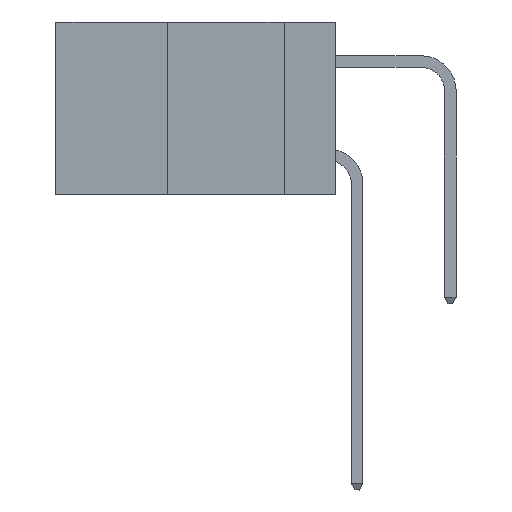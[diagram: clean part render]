
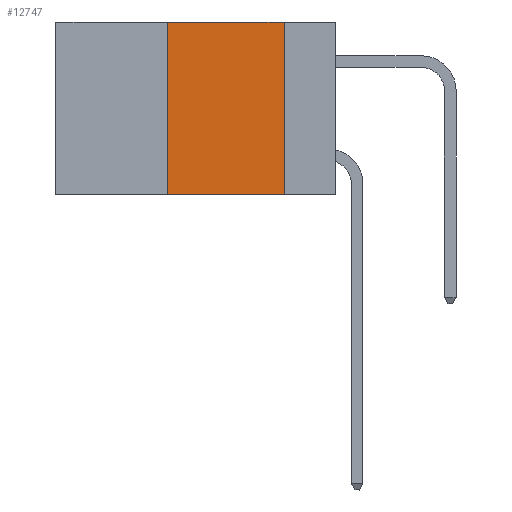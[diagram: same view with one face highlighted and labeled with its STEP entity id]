
A CAD part, left-side view. The second image highlights one B-rep face of the part: STEP entity #12747.
In plain terms, the highlighted planar face has unit normal (-1, 0, 0).
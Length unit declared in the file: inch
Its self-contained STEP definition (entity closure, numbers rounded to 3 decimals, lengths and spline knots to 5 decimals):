
#814 = CARTESIAN_POINT ( 'NONE',  ( 0., 0.36, 0. ) ) ;
#1652 = DIRECTION ( 'NONE',  ( 1., 0., 0. ) ) ;
#2081 = DIRECTION ( 'NONE',  ( 0., 0., 1. ) ) ;
#2251 = VERTEX_POINT ( 'NONE', #4173 ) ;
#2275 = EDGE_CURVE ( 'NONE', #2251, #18373, #2592, .T. ) ;
#2592 = LINE ( 'NONE', #14858, #3052 ) ;
#3052 = VECTOR ( 'NONE', #22942, 39.37008 ) ;
#3455 = AXIS2_PLACEMENT_3D ( 'NONE', #15916, #1652, #4041 ) ;
#3815 = CARTESIAN_POINT ( 'NONE',  ( 0., 0.11, -0.37 ) ) ;
#4041 = DIRECTION ( 'NONE',  ( 0., 0., -1. ) ) ;
#4173 = CARTESIAN_POINT ( 'NONE',  ( 0., 0.11, 0. ) ) ;
#4659 = CARTESIAN_POINT ( 'NONE',  ( 0., 0.6, 0. ) ) ;
#5671 = VERTEX_POINT ( 'NONE', #814 ) ;
#5960 = CARTESIAN_POINT ( 'NONE',  ( 0., 0.36, -0.37 ) ) ;
#6097 = ORIENTED_EDGE ( 'NONE', *, *, #25650, .T. ) ;
#7870 = FACE_OUTER_BOUND ( 'NONE', #7957, .T. ) ;
#7957 = EDGE_LOOP ( 'NONE', ( #19853, #11648, #8887, #6097 ) ) ;
#8023 = LINE ( 'NONE', #13959, #14735 ) ;
#8887 = ORIENTED_EDGE ( 'NONE', *, *, #11082, .F. ) ;
#9307 = EDGE_CURVE ( 'NONE', #5671, #2251, #21019, .T. ) ;
#11082 = EDGE_CURVE ( 'NONE', #20984, #5671, #8023, .T. ) ;
#11648 = ORIENTED_EDGE ( 'NONE', *, *, #9307, .F. ) ;
#12092 = PLANE ( 'NONE',  #3455 ) ;
#12110 = CARTESIAN_POINT ( 'NONE',  ( 0., 0.6, -0.37 ) ) ;
#12747 = ADVANCED_FACE ( 'NONE', ( #7870 ), #12092, .F. ) ;
#13959 = CARTESIAN_POINT ( 'NONE',  ( 0., 0.36, 0. ) ) ;
#14329 = DIRECTION ( 'NONE',  ( 0., -1., 0. ) ) ;
#14735 = VECTOR ( 'NONE', #2081, 39.37008 ) ;
#14858 = CARTESIAN_POINT ( 'NONE',  ( 0., 0.11, 0. ) ) ;
#15106 = VECTOR ( 'NONE', #24860, 39.37008 ) ;
#15916 = CARTESIAN_POINT ( 'NONE',  ( 0., 0.6, 0. ) ) ;
#16063 = LINE ( 'NONE', #12110, #25809 ) ;
#18373 = VERTEX_POINT ( 'NONE', #3815 ) ;
#19853 = ORIENTED_EDGE ( 'NONE', *, *, #2275, .F. ) ;
#20984 = VERTEX_POINT ( 'NONE', #5960 ) ;
#21019 = LINE ( 'NONE', #4659, #15106 ) ;
#22942 = DIRECTION ( 'NONE',  ( 0., 0., -1. ) ) ;
#24860 = DIRECTION ( 'NONE',  ( 0., -1., 0. ) ) ;
#25650 = EDGE_CURVE ( 'NONE', #20984, #18373, #16063, .T. ) ;
#25809 = VECTOR ( 'NONE', #14329, 39.37008 ) ;
